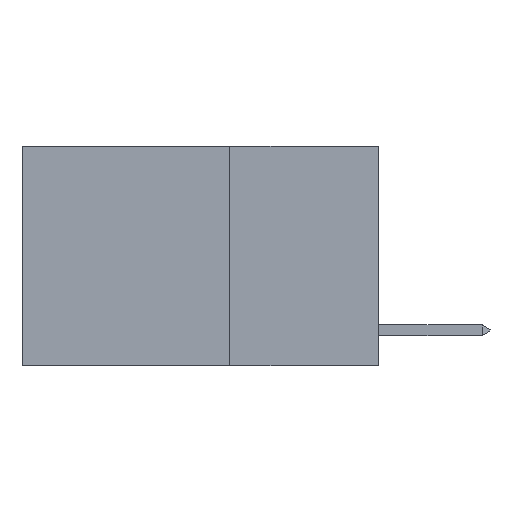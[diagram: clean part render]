
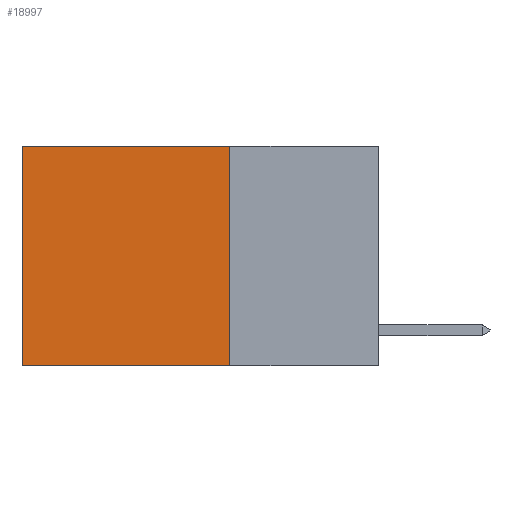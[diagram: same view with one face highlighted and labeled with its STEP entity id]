
A CAD part, left-side view. The second image highlights one B-rep face of the part: STEP entity #18997.
In plain terms, the highlighted planar face has unit normal (-1, 0, 0).
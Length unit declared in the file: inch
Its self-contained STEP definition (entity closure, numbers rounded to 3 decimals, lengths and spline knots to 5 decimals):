
#283 = LINE ( 'NONE', #20575, #13970 ) ;
#538 = CARTESIAN_POINT ( 'NONE',  ( 0.2625, 0.25, 0. ) ) ;
#2093 = DIRECTION ( 'NONE',  ( 0., 0., -1. ) ) ;
#2213 = LINE ( 'NONE', #9022, #19846 ) ;
#2938 = EDGE_CURVE ( 'NONE', #21337, #16282, #5035, .T. ) ;
#4223 = VECTOR ( 'NONE', #7932, 39.37008 ) ;
#4794 = CARTESIAN_POINT ( 'NONE',  ( 0.2625, 0.6, 0. ) ) ;
#4923 = DIRECTION ( 'NONE',  ( 0., 1., 0. ) ) ;
#5035 = LINE ( 'NONE', #14976, #7159 ) ;
#5335 = DIRECTION ( 'NONE',  ( 1., 0., 0. ) ) ;
#5657 = PLANE ( 'NONE',  #18711 ) ;
#5768 = EDGE_CURVE ( 'NONE', #16254, #21337, #283, .T. ) ;
#7029 = CARTESIAN_POINT ( 'NONE',  ( 0.2625, 0.25, 0. ) ) ;
#7159 = VECTOR ( 'NONE', #4923, 39.37008 ) ;
#7558 = DIRECTION ( 'NONE',  ( 0., 1., 0. ) ) ;
#7932 = DIRECTION ( 'NONE',  ( 0., 0., -1. ) ) ;
#7982 = ORIENTED_EDGE ( 'NONE', *, *, #16501, .T. ) ;
#9022 = CARTESIAN_POINT ( 'NONE',  ( 0.2625, 0.25, 0. ) ) ;
#11489 = LINE ( 'NONE', #20298, #4223 ) ;
#11494 = ORIENTED_EDGE ( 'NONE', *, *, #2938, .F. ) ;
#12152 = CARTESIAN_POINT ( 'NONE',  ( 0.2625, 0.25, -0.37 ) ) ;
#12387 = CARTESIAN_POINT ( 'NONE',  ( 0.2625, 0.6, -0.37 ) ) ;
#12916 = EDGE_LOOP ( 'NONE', ( #7982, #11494, #17163, #16409 ) ) ;
#13970 = VECTOR ( 'NONE', #15234, 39.37008 ) ;
#14976 = CARTESIAN_POINT ( 'NONE',  ( 0.2625, 0.25, -0.37 ) ) ;
#14992 = EDGE_CURVE ( 'NONE', #16254, #18880, #2213, .T. ) ;
#15234 = DIRECTION ( 'NONE',  ( 0., 0., -1. ) ) ;
#16254 = VERTEX_POINT ( 'NONE', #7029 ) ;
#16282 = VERTEX_POINT ( 'NONE', #12387 ) ;
#16409 = ORIENTED_EDGE ( 'NONE', *, *, #14992, .T. ) ;
#16501 = EDGE_CURVE ( 'NONE', #18880, #16282, #11489, .T. ) ;
#17163 = ORIENTED_EDGE ( 'NONE', *, *, #5768, .F. ) ;
#17262 = FACE_OUTER_BOUND ( 'NONE', #12916, .T. ) ;
#18711 = AXIS2_PLACEMENT_3D ( 'NONE', #538, #5335, #2093 ) ;
#18880 = VERTEX_POINT ( 'NONE', #4794 ) ;
#18997 = ADVANCED_FACE ( 'NONE', ( #17262 ), #5657, .F. ) ;
#19846 = VECTOR ( 'NONE', #7558, 39.37008 ) ;
#20298 = CARTESIAN_POINT ( 'NONE',  ( 0.2625, 0.6, 0. ) ) ;
#20575 = CARTESIAN_POINT ( 'NONE',  ( 0.2625, 0.25, 0. ) ) ;
#21337 = VERTEX_POINT ( 'NONE', #12152 ) ;
